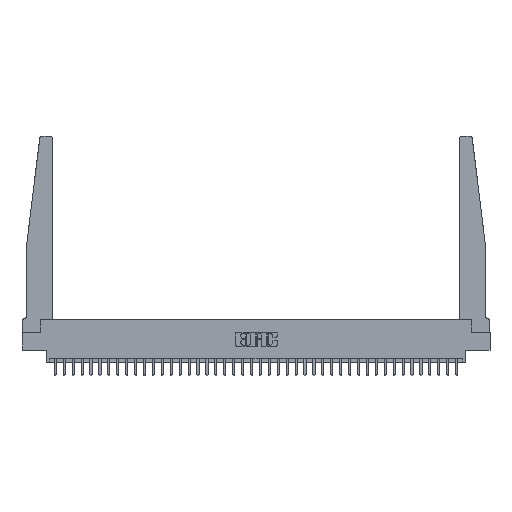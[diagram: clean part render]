
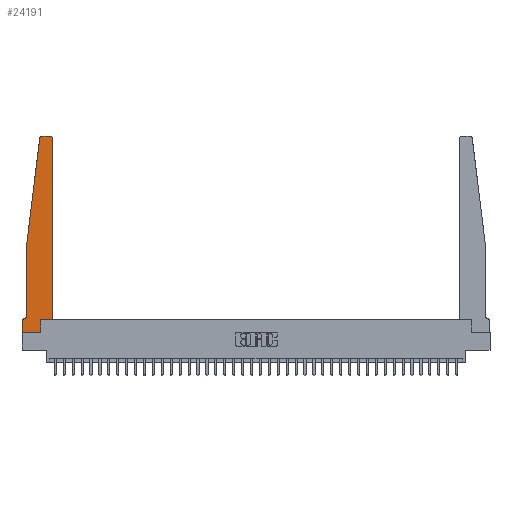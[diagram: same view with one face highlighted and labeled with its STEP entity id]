
A CAD part, top view. The second image highlights one B-rep face of the part: STEP entity #24191.
In plain terms, the highlighted planar face has unit normal (0, 0, 1).
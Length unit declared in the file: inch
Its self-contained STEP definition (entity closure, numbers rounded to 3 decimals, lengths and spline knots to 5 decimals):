
#552 = VECTOR ( 'NONE', #24507, 39.37008 ) ;
#559 = CARTESIAN_POINT ( 'NONE',  ( 0., 0.1875, 0.37 ) ) ;
#932 = CIRCLE ( 'NONE', #27557, 0.03 ) ;
#989 = DIRECTION ( 'NONE',  ( 0., 0., 1. ) ) ;
#1539 = CARTESIAN_POINT ( 'NONE',  ( 0.065, 1.25, 0.37 ) ) ;
#1760 = EDGE_CURVE ( 'NONE', #27935, #2618, #10325, .T. ) ;
#1809 = AXIS2_PLACEMENT_3D ( 'NONE', #18179, #28977, #20663 ) ;
#1855 = CARTESIAN_POINT ( 'NONE',  ( 0.25, 2.75, 0.37 ) ) ;
#2618 = VERTEX_POINT ( 'NONE', #21513 ) ;
#2696 = VERTEX_POINT ( 'NONE', #20081 ) ;
#2825 = CARTESIAN_POINT ( 'NONE',  ( 0.2605, 0.18, 0.37 ) ) ;
#2871 = VERTEX_POINT ( 'NONE', #28906 ) ;
#3695 = VERTEX_POINT ( 'NONE', #16986 ) ;
#4683 = ORIENTED_EDGE ( 'NONE', *, *, #31542, .T. ) ;
#4751 = DIRECTION ( 'NONE',  ( -0.122, -0.992, 0. ) ) ;
#5046 = EDGE_CURVE ( 'NONE', #3695, #25564, #16727, .T. ) ;
#5106 = DIRECTION ( 'NONE',  ( 0., 1., 0. ) ) ;
#6308 = LINE ( 'NONE', #1539, #22182 ) ;
#6418 = CARTESIAN_POINT ( 'NONE',  ( 0., 0., 0.37 ) ) ;
#7841 = AXIS2_PLACEMENT_3D ( 'NONE', #10240, #21040, #18227 ) ;
#8289 = CARTESIAN_POINT ( 'NONE',  ( 0.425, 0.18, 0.37 ) ) ;
#8475 = DIRECTION ( 'NONE',  ( 1., 0., 0. ) ) ;
#8706 = ORIENTED_EDGE ( 'NONE', *, *, #18037, .T. ) ;
#8712 = ORIENTED_EDGE ( 'NONE', *, *, #16273, .T. ) ;
#8791 = EDGE_CURVE ( 'NONE', #31720, #2871, #32743, .T. ) ;
#9723 = CIRCLE ( 'NONE', #1809, 0.03 ) ;
#10086 = VECTOR ( 'NONE', #16108, 39.37008 ) ;
#10240 = CARTESIAN_POINT ( 'NONE',  ( 0.015, 0.2375, 0.37 ) ) ;
#10325 = LINE ( 'NONE', #1855, #18374 ) ;
#10327 = ORIENTED_EDGE ( 'NONE', *, *, #5046, .T. ) ;
#10475 = CARTESIAN_POINT ( 'NONE',  ( 0.425, 0.18, 0.37 ) ) ;
#11485 = VERTEX_POINT ( 'NONE', #10475 ) ;
#11994 = VERTEX_POINT ( 'NONE', #14669 ) ;
#12015 = CARTESIAN_POINT ( 'NONE',  ( 0., 0., 0.37 ) ) ;
#12260 = EDGE_CURVE ( 'NONE', #25564, #31909, #23868, .T. ) ;
#12701 = DIRECTION ( 'NONE',  ( 1., 0., 0. ) ) ;
#13184 = CARTESIAN_POINT ( 'NONE',  ( 0.2605, 0., 0.37 ) ) ;
#13187 = EDGE_CURVE ( 'NONE', #20882, #3695, #22006, .T. ) ;
#13690 = CARTESIAN_POINT ( 'NONE',  ( 0.065, 0.2375, 0.37 ) ) ;
#13790 = LINE ( 'NONE', #24250, #10086 ) ;
#14157 = CARTESIAN_POINT ( 'NONE',  ( 0.425, 0.18, 0.37 ) ) ;
#14206 = ORIENTED_EDGE ( 'NONE', *, *, #28389, .T. ) ;
#14669 = CARTESIAN_POINT ( 'NONE',  ( 0.425, 2.72, 0.37 ) ) ;
#15563 = CARTESIAN_POINT ( 'NONE',  ( 0., 0.1875, 0.37 ) ) ;
#15656 = DIRECTION ( 'NONE',  ( -1., 0., 0. ) ) ;
#15713 = CARTESIAN_POINT ( 'NONE',  ( 0.065, 1.25, 0.37 ) ) ;
#16108 = DIRECTION ( 'NONE',  ( -1., 0., 0. ) ) ;
#16273 = EDGE_CURVE ( 'NONE', #2871, #20882, #13790, .T. ) ;
#16314 = EDGE_CURVE ( 'NONE', #11485, #11994, #27267, .T. ) ;
#16470 = CARTESIAN_POINT ( 'NONE',  ( 0.395, 2.75, 0.37 ) ) ;
#16727 = LINE ( 'NONE', #6418, #22190 ) ;
#16929 = DIRECTION ( 'NONE',  ( 1., 0., 0. ) ) ;
#16986 = CARTESIAN_POINT ( 'NONE',  ( 0., 0., 0.37 ) ) ;
#17414 = DIRECTION ( 'NONE',  ( 1., 0., 0. ) ) ;
#17869 = DIRECTION ( 'NONE',  ( 0., 0., 1. ) ) ;
#18037 = EDGE_CURVE ( 'NONE', #2696, #25596, #26694, .T. ) ;
#18179 = CARTESIAN_POINT ( 'NONE',  ( 0.395, 2.72, 0.37 ) ) ;
#18227 = DIRECTION ( 'NONE',  ( -1., 0., 0. ) ) ;
#18374 = VECTOR ( 'NONE', #15656, 39.37008 ) ;
#18990 = ORIENTED_EDGE ( 'NONE', *, *, #27949, .T. ) ;
#19104 = DIRECTION ( 'NONE',  ( 0., 1., 0. ) ) ;
#19393 = EDGE_LOOP ( 'NONE', ( #32698, #23459, #8706, #14206, #25638, #8712, #27461, #10327, #29041, #18990, #24754, #4683 ) ) ;
#19945 = EDGE_CURVE ( 'NONE', #2618, #2696, #932, .T. ) ;
#20081 = CARTESIAN_POINT ( 'NONE',  ( 0.24675, 2.72367, 0.37 ) ) ;
#20663 = DIRECTION ( 'NONE',  ( 1., 0., 0. ) ) ;
#20882 = VERTEX_POINT ( 'NONE', #559 ) ;
#21040 = DIRECTION ( 'NONE',  ( 0., 0., -1. ) ) ;
#21352 = VECTOR ( 'NONE', #5106, 39.37008 ) ;
#21513 = CARTESIAN_POINT ( 'NONE',  ( 0.27653, 2.75, 0.37 ) ) ;
#22006 = LINE ( 'NONE', #12015, #552 ) ;
#22134 = LINE ( 'NONE', #14157, #27275 ) ;
#22182 = VECTOR ( 'NONE', #23127, 39.37008 ) ;
#22190 = VECTOR ( 'NONE', #17414, 39.37008 ) ;
#22417 = CARTESIAN_POINT ( 'NONE',  ( 0.27653, 2.72, 0.37 ) ) ;
#22993 = PLANE ( 'NONE',  #26040 ) ;
#23127 = DIRECTION ( 'NONE',  ( 0., -1., 0. ) ) ;
#23459 = ORIENTED_EDGE ( 'NONE', *, *, #19945, .T. ) ;
#23868 = LINE ( 'NONE', #2825, #21352 ) ;
#24013 = VECTOR ( 'NONE', #4751, 39.37008 ) ;
#24191 = ADVANCED_FACE ( 'NONE', ( #28504 ), #22993, .T. ) ;
#24250 = CARTESIAN_POINT ( 'NONE',  ( 0.065, 0.1875, 0.37 ) ) ;
#24507 = DIRECTION ( 'NONE',  ( 0., -1., 0. ) ) ;
#24754 = ORIENTED_EDGE ( 'NONE', *, *, #16314, .T. ) ;
#25564 = VERTEX_POINT ( 'NONE', #13184 ) ;
#25596 = VERTEX_POINT ( 'NONE', #33181 ) ;
#25638 = ORIENTED_EDGE ( 'NONE', *, *, #8791, .T. ) ;
#26040 = AXIS2_PLACEMENT_3D ( 'NONE', #15563, #17869, #12701 ) ;
#26694 = LINE ( 'NONE', #15713, #24013 ) ;
#27267 = LINE ( 'NONE', #8289, #29881 ) ;
#27275 = VECTOR ( 'NONE', #8475, 39.37008 ) ;
#27461 = ORIENTED_EDGE ( 'NONE', *, *, #13187, .T. ) ;
#27557 = AXIS2_PLACEMENT_3D ( 'NONE', #22417, #989, #16929 ) ;
#27935 = VERTEX_POINT ( 'NONE', #16470 ) ;
#27949 = EDGE_CURVE ( 'NONE', #31909, #11485, #22134, .T. ) ;
#28389 = EDGE_CURVE ( 'NONE', #25596, #31720, #6308, .T. ) ;
#28504 = FACE_OUTER_BOUND ( 'NONE', #19393, .T. ) ;
#28906 = CARTESIAN_POINT ( 'NONE',  ( 0.015, 0.1875, 0.37 ) ) ;
#28977 = DIRECTION ( 'NONE',  ( 0., 0., 1. ) ) ;
#29041 = ORIENTED_EDGE ( 'NONE', *, *, #12260, .T. ) ;
#29881 = VECTOR ( 'NONE', #19104, 39.37008 ) ;
#31542 = EDGE_CURVE ( 'NONE', #11994, #27935, #9723, .T. ) ;
#31720 = VERTEX_POINT ( 'NONE', #13690 ) ;
#31909 = VERTEX_POINT ( 'NONE', #34210 ) ;
#32698 = ORIENTED_EDGE ( 'NONE', *, *, #1760, .T. ) ;
#32743 = CIRCLE ( 'NONE', #7841, 0.05 ) ;
#33181 = CARTESIAN_POINT ( 'NONE',  ( 0.065, 1.25, 0.37 ) ) ;
#34210 = CARTESIAN_POINT ( 'NONE',  ( 0.2605, 0.18, 0.37 ) ) ;
